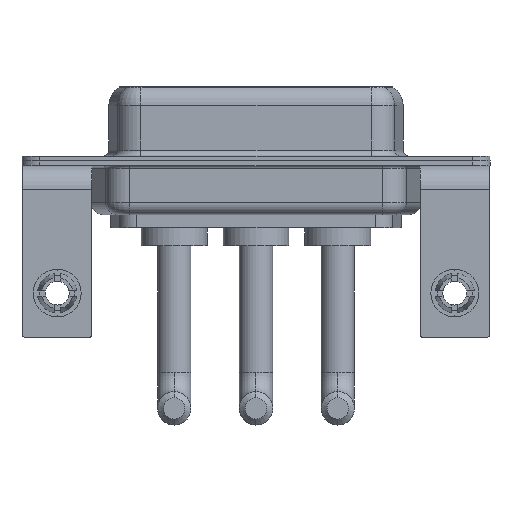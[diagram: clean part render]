
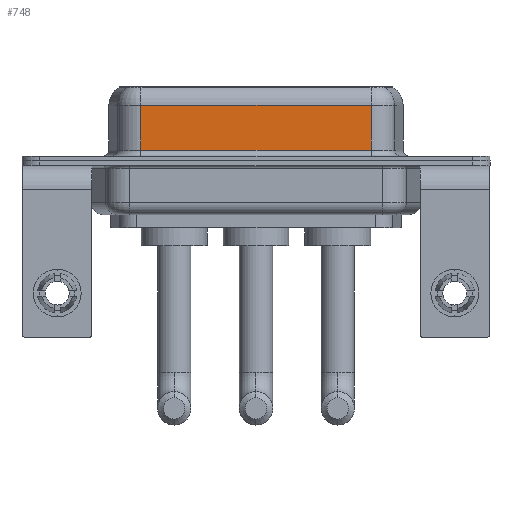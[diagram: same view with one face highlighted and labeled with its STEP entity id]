
A CAD part, front view. The second image highlights one B-rep face of the part: STEP entity #748.
In plain terms, the highlighted planar face has unit normal (0, -1, 0).
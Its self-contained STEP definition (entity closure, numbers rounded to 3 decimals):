
#291 = DIRECTION ( 'NONE',  ( 0., 0., -1. ) ) ;
#406 = CARTESIAN_POINT ( 'NONE',  ( 26.287, -3.95, 6.4 ) ) ;
#583 = CARTESIAN_POINT ( 'NONE',  ( 26.287, -3.95, 0.9 ) ) ;
#748 = ADVANCED_FACE ( 'NONE', ( #5843 ), #13901, .F. ) ;
#857 = VECTOR ( 'NONE', #8761, 1000. ) ;
#1413 = EDGE_CURVE ( 'NONE', #2674, #8625, #5129, .T. ) ;
#1455 = DIRECTION ( 'NONE',  ( 0., 1., 0. ) ) ;
#1678 = VECTOR ( 'NONE', #4019, 1000. ) ;
#1926 = CARTESIAN_POINT ( 'NONE',  ( 26.287, -3.95, 6.4 ) ) ;
#1957 = CARTESIAN_POINT ( 'NONE',  ( 26.287, -3.95, 4.65 ) ) ;
#1979 = LINE ( 'NONE', #13155, #857 ) ;
#2142 = VERTEX_POINT ( 'NONE', #8369 ) ;
#2275 = ORIENTED_EDGE ( 'NONE', *, *, #1413, .F. ) ;
#2674 = VERTEX_POINT ( 'NONE', #1957 ) ;
#2725 = CARTESIAN_POINT ( 'NONE',  ( 7.013, -3.95, 6.4 ) ) ;
#3955 = VECTOR ( 'NONE', #291, 1000. ) ;
#4019 = DIRECTION ( 'NONE',  ( 0., 0., -1. ) ) ;
#5129 = LINE ( 'NONE', #1926, #1678 ) ;
#5181 = LINE ( 'NONE', #12921, #12998 ) ;
#5688 = ORIENTED_EDGE ( 'NONE', *, *, #10892, .T. ) ;
#5843 = FACE_OUTER_BOUND ( 'NONE', #14084, .T. ) ;
#6507 = CARTESIAN_POINT ( 'NONE',  ( 7.013, -3.95, 0.9 ) ) ;
#8369 = CARTESIAN_POINT ( 'NONE',  ( 7.013, -3.95, 4.65 ) ) ;
#8440 = DIRECTION ( 'NONE',  ( 1., 0., 0. ) ) ;
#8625 = VERTEX_POINT ( 'NONE', #583 ) ;
#8674 = ORIENTED_EDGE ( 'NONE', *, *, #10032, .T. ) ;
#8761 = DIRECTION ( 'NONE',  ( -1., 0., 0. ) ) ;
#9054 = AXIS2_PLACEMENT_3D ( 'NONE', #406, #1455, #9202 ) ;
#9202 = DIRECTION ( 'NONE',  ( 0., 0., 1. ) ) ;
#10032 = EDGE_CURVE ( 'NONE', #10195, #8625, #5181, .T. ) ;
#10195 = VERTEX_POINT ( 'NONE', #6507 ) ;
#10700 = ORIENTED_EDGE ( 'NONE', *, *, #10990, .T. ) ;
#10892 = EDGE_CURVE ( 'NONE', #2142, #10195, #14069, .T. ) ;
#10990 = EDGE_CURVE ( 'NONE', #2674, #2142, #1979, .T. ) ;
#12921 = CARTESIAN_POINT ( 'NONE',  ( 26.287, -3.95, 0.9 ) ) ;
#12998 = VECTOR ( 'NONE', #8440, 1000. ) ;
#13155 = CARTESIAN_POINT ( 'NONE',  ( 26.287, -3.95, 4.65 ) ) ;
#13901 = PLANE ( 'NONE',  #9054 ) ;
#14069 = LINE ( 'NONE', #2725, #3955 ) ;
#14084 = EDGE_LOOP ( 'NONE', ( #2275, #10700, #5688, #8674 ) ) ;
